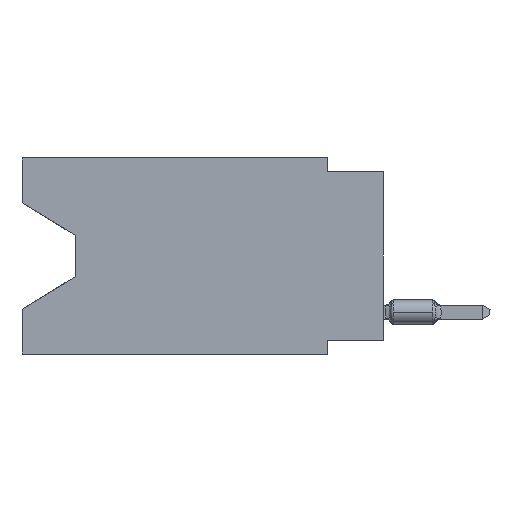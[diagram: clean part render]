
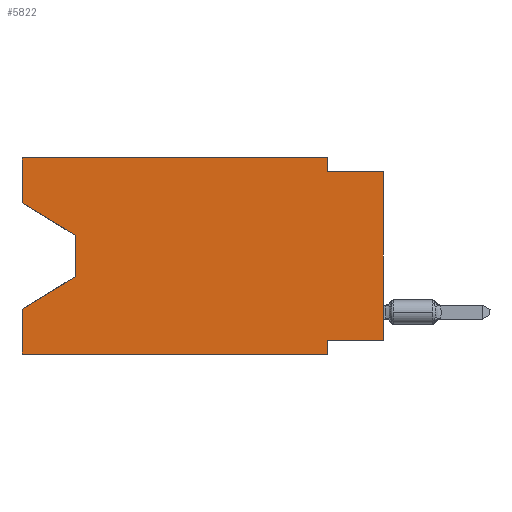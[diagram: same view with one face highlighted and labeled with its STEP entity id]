
A CAD part, left-side view. The second image highlights one B-rep face of the part: STEP entity #5822.
In plain terms, the highlighted planar face has unit normal (-1, 0, 0).
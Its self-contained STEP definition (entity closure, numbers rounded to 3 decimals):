
#74 = VECTOR ( 'NONE', #22205, 1000. ) ;
#884 = VECTOR ( 'NONE', #17402, 1000. ) ;
#1864 = VERTEX_POINT ( 'NONE', #2160 ) ;
#1986 = EDGE_CURVE ( 'NONE', #20144, #10266, #3345, .T. ) ;
#2160 = CARTESIAN_POINT ( 'NONE',  ( 0., 13.97, -5.385 ) ) ;
#2673 = CARTESIAN_POINT ( 'NONE',  ( 0., 0., -8.255 ) ) ;
#2850 = EDGE_CURVE ( 'NONE', #20144, #5787, #25452, .T. ) ;
#2931 = PLANE ( 'NONE',  #22679 ) ;
#3345 = LINE ( 'NONE', #17653, #74 ) ;
#3395 = CARTESIAN_POINT ( 'NONE',  ( 0., 16.383, -8.89 ) ) ;
#3841 = EDGE_CURVE ( 'NONE', #13593, #8445, #21917, .T. ) ;
#4242 = LINE ( 'NONE', #8260, #20286 ) ;
#4644 = CARTESIAN_POINT ( 'NONE',  ( 0., 16.383, 0. ) ) ;
#4666 = LINE ( 'NONE', #4925, #6723 ) ;
#4925 = CARTESIAN_POINT ( 'NONE',  ( 0., 16.383, -2.038 ) ) ;
#4988 = DIRECTION ( 'NONE',  ( 0., 1., 0. ) ) ;
#5302 = VECTOR ( 'NONE', #22264, 1000. ) ;
#5313 = DIRECTION ( 'NONE',  ( 0., 0., -1. ) ) ;
#5427 = VERTEX_POINT ( 'NONE', #13412 ) ;
#5440 = EDGE_CURVE ( 'NONE', #22048, #20773, #4666, .T. ) ;
#5758 = LINE ( 'NONE', #26831, #23807 ) ;
#5787 = VERTEX_POINT ( 'NONE', #14879 ) ;
#5822 = ADVANCED_FACE ( 'NONE', ( #7220 ), #2931, .F. ) ;
#6302 = ORIENTED_EDGE ( 'NONE', *, *, #14123, .T. ) ;
#6312 = CARTESIAN_POINT ( 'NONE',  ( 0., 13.97, -5.385 ) ) ;
#6635 = ORIENTED_EDGE ( 'NONE', *, *, #5440, .T. ) ;
#6723 = VECTOR ( 'NONE', #21579, 1000. ) ;
#6922 = EDGE_CURVE ( 'NONE', #18702, #6981, #10197, .T. ) ;
#6979 = ORIENTED_EDGE ( 'NONE', *, *, #6922, .F. ) ;
#6981 = VERTEX_POINT ( 'NONE', #27370 ) ;
#7220 = FACE_OUTER_BOUND ( 'NONE', #9575, .T. ) ;
#8260 = CARTESIAN_POINT ( 'NONE',  ( 0., 0., 0. ) ) ;
#8305 = EDGE_CURVE ( 'NONE', #5427, #17777, #21422, .T. ) ;
#8443 = ORIENTED_EDGE ( 'NONE', *, *, #20374, .T. ) ;
#8445 = VERTEX_POINT ( 'NONE', #19017 ) ;
#9040 = CARTESIAN_POINT ( 'NONE',  ( 0., 16.383, 0. ) ) ;
#9176 = DIRECTION ( 'NONE',  ( 1., 0., 0. ) ) ;
#9575 = EDGE_LOOP ( 'NONE', ( #6635, #6302, #8443, #19063, #19405, #25220, #12319, #20617, #6979, #16933, #26650, #19790 ) ) ;
#9982 = VECTOR ( 'NONE', #19354, 1000. ) ;
#10197 = LINE ( 'NONE', #20860, #12562 ) ;
#10266 = VERTEX_POINT ( 'NONE', #16454 ) ;
#10310 = CARTESIAN_POINT ( 'NONE',  ( 0., 2.54, -0.635 ) ) ;
#10762 = LINE ( 'NONE', #6312, #9982 ) ;
#12319 = ORIENTED_EDGE ( 'NONE', *, *, #3841, .F. ) ;
#12397 = VECTOR ( 'NONE', #25586, 1000. ) ;
#12562 = VECTOR ( 'NONE', #18934, 1000. ) ;
#13412 = CARTESIAN_POINT ( 'NONE',  ( 0., 16.383, 0. ) ) ;
#13593 = VERTEX_POINT ( 'NONE', #2673 ) ;
#13711 = CARTESIAN_POINT ( 'NONE',  ( 0., 2.54, 0. ) ) ;
#13828 = CARTESIAN_POINT ( 'NONE',  ( 0., 2.54, 0. ) ) ;
#14123 = EDGE_CURVE ( 'NONE', #20773, #1864, #5758, .T. ) ;
#14216 = EDGE_CURVE ( 'NONE', #13593, #6981, #4242, .T. ) ;
#14746 = CARTESIAN_POINT ( 'NONE',  ( 0., 13.97, -3.505 ) ) ;
#14879 = CARTESIAN_POINT ( 'NONE',  ( 0., 2.54, -8.89 ) ) ;
#15062 = EDGE_CURVE ( 'NONE', #22048, #5427, #20942, .T. ) ;
#15705 = EDGE_CURVE ( 'NONE', #17777, #18702, #16045, .T. ) ;
#15823 = DIRECTION ( 'NONE',  ( 0., 0., -1. ) ) ;
#16045 = LINE ( 'NONE', #13828, #5302 ) ;
#16454 = CARTESIAN_POINT ( 'NONE',  ( 0., 16.383, -6.852 ) ) ;
#16785 = DIRECTION ( 'NONE',  ( 0., 0., 1. ) ) ;
#16854 = DIRECTION ( 'NONE',  ( 0., 0., 1. ) ) ;
#16855 = VECTOR ( 'NONE', #4988, 1000. ) ;
#16933 = ORIENTED_EDGE ( 'NONE', *, *, #15705, .F. ) ;
#17402 = DIRECTION ( 'NONE',  ( 0., -1., 0. ) ) ;
#17616 = VECTOR ( 'NONE', #16785, 1000. ) ;
#17653 = CARTESIAN_POINT ( 'NONE',  ( 0., 16.383, 0. ) ) ;
#17777 = VERTEX_POINT ( 'NONE', #13711 ) ;
#18702 = VERTEX_POINT ( 'NONE', #10310 ) ;
#18934 = DIRECTION ( 'NONE',  ( 0., -1., 0. ) ) ;
#19017 = CARTESIAN_POINT ( 'NONE',  ( 0., 2.54, -8.255 ) ) ;
#19063 = ORIENTED_EDGE ( 'NONE', *, *, #1986, .F. ) ;
#19354 = DIRECTION ( 'NONE',  ( 0., 0.855, -0.519 ) ) ;
#19405 = ORIENTED_EDGE ( 'NONE', *, *, #2850, .T. ) ;
#19698 = DIRECTION ( 'NONE',  ( 0., 0., -1. ) ) ;
#19778 = LINE ( 'NONE', #22379, #23165 ) ;
#19790 = ORIENTED_EDGE ( 'NONE', *, *, #15062, .F. ) ;
#20144 = VERTEX_POINT ( 'NONE', #3395 ) ;
#20286 = VECTOR ( 'NONE', #16854, 1000. ) ;
#20374 = EDGE_CURVE ( 'NONE', #1864, #10266, #10762, .T. ) ;
#20617 = ORIENTED_EDGE ( 'NONE', *, *, #14216, .T. ) ;
#20773 = VERTEX_POINT ( 'NONE', #14746 ) ;
#20860 = CARTESIAN_POINT ( 'NONE',  ( 0., 0., -0.635 ) ) ;
#20942 = LINE ( 'NONE', #27312, #17616 ) ;
#21422 = LINE ( 'NONE', #4644, #884 ) ;
#21579 = DIRECTION ( 'NONE',  ( 0., -0.855, -0.519 ) ) ;
#21917 = LINE ( 'NONE', #23992, #16855 ) ;
#22048 = VERTEX_POINT ( 'NONE', #23753 ) ;
#22205 = DIRECTION ( 'NONE',  ( 0., 0., 1. ) ) ;
#22264 = DIRECTION ( 'NONE',  ( 0., 0., -1. ) ) ;
#22379 = CARTESIAN_POINT ( 'NONE',  ( 0., 2.54, -8.89 ) ) ;
#22679 = AXIS2_PLACEMENT_3D ( 'NONE', #9040, #9176, #15823 ) ;
#23165 = VECTOR ( 'NONE', #5313, 1000. ) ;
#23753 = CARTESIAN_POINT ( 'NONE',  ( 0., 16.383, -2.038 ) ) ;
#23807 = VECTOR ( 'NONE', #19698, 1000. ) ;
#23992 = CARTESIAN_POINT ( 'NONE',  ( 0., 0., -8.255 ) ) ;
#25220 = ORIENTED_EDGE ( 'NONE', *, *, #26386, .F. ) ;
#25452 = LINE ( 'NONE', #25722, #12397 ) ;
#25586 = DIRECTION ( 'NONE',  ( 0., -1., 0. ) ) ;
#25722 = CARTESIAN_POINT ( 'NONE',  ( 0., 16.383, -8.89 ) ) ;
#26386 = EDGE_CURVE ( 'NONE', #8445, #5787, #19778, .T. ) ;
#26650 = ORIENTED_EDGE ( 'NONE', *, *, #8305, .F. ) ;
#26831 = CARTESIAN_POINT ( 'NONE',  ( 0., 13.97, -3.505 ) ) ;
#27312 = CARTESIAN_POINT ( 'NONE',  ( 0., 16.383, 0. ) ) ;
#27370 = CARTESIAN_POINT ( 'NONE',  ( 0., 0., -0.635 ) ) ;
